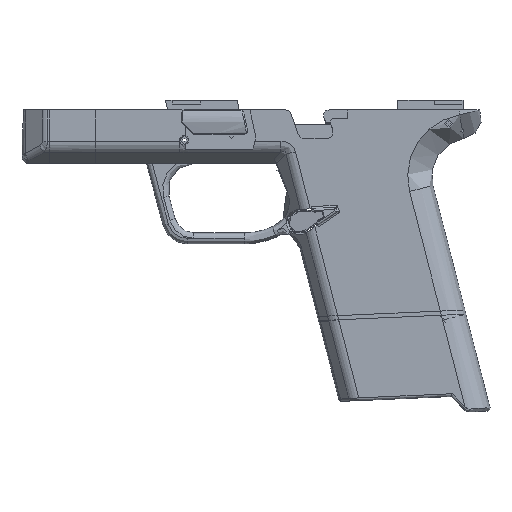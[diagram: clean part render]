
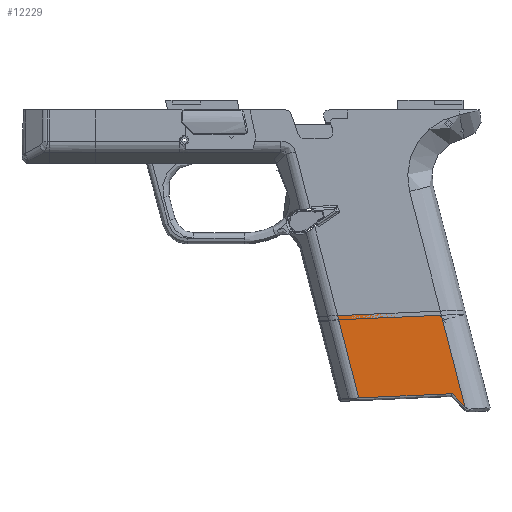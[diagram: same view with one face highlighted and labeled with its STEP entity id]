
A CAD part, left-side view. The second image highlights one B-rep face of the part: STEP entity #12229.
In plain terms, the highlighted face is planar.
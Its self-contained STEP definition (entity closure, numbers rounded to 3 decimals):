
#959=PLANE('',#13436);
#1609=FACE_OUTER_BOUND('',#2307,.T.);
#2307=EDGE_LOOP('',(#11234,#11235,#11236,#11237,#11238));
#3367=LINE('',#23857,#4460);
#3374=LINE('',#23978,#4467);
#3386=LINE('',#24009,#4479);
#3387=LINE('',#24013,#4480);
#3388=LINE('',#24014,#4481);
#4460=VECTOR('',#16590,10.);
#4467=VECTOR('',#16637,10.);
#4479=VECTOR('',#16671,10.);
#4480=VECTOR('',#16676,10.);
#4481=VECTOR('',#16677,10.);
#5935=VERTEX_POINT('',#23689);
#5946=VERTEX_POINT('',#23856);
#5960=VERTEX_POINT('',#23973);
#5968=VERTEX_POINT('',#24008);
#5969=VERTEX_POINT('',#24012);
#7700=EDGE_CURVE('',#5935,#5946,#3367,.T.);
#7723=EDGE_CURVE('',#5946,#5960,#3374,.T.);
#7738=EDGE_CURVE('',#5968,#5960,#3386,.T.);
#7740=EDGE_CURVE('',#5969,#5935,#3387,.T.);
#7741=EDGE_CURVE('',#5969,#5968,#3388,.T.);
#11234=ORIENTED_EDGE('',*,*,#7723,.F.);
#11235=ORIENTED_EDGE('',*,*,#7700,.F.);
#11236=ORIENTED_EDGE('',*,*,#7740,.F.);
#11237=ORIENTED_EDGE('',*,*,#7741,.T.);
#11238=ORIENTED_EDGE('',*,*,#7738,.T.);
#12229=ADVANCED_FACE('',(#1609),#959,.T.);
#13436=AXIS2_PLACEMENT_3D('',#24011,#16674,#16675);
#16590=DIRECTION('',(0.,0.697,-0.717));
#16637=DIRECTION('',(0.,0.999,0.044));
#16671=DIRECTION('',(0.,-0.249,0.969));
#16674=DIRECTION('center_axis',(1.,0.,0.));
#16675=DIRECTION('ref_axis',(0.,0.999,0.044));
#16676=DIRECTION('',(0.,-0.249,0.969));
#16677=DIRECTION('',(0.,0.999,0.044));
#23689=CARTESIAN_POINT('',(22.175,-83.249,100.107));
#23856=CARTESIAN_POINT('',(22.175,-78.67,95.402));
#23857=CARTESIAN_POINT('',(22.175,-73.025,89.603));
#23973=CARTESIAN_POINT('',(22.175,-44.727,96.906));
#23978=CARTESIAN_POINT('',(22.175,-44.598,96.911));
#24008=CARTESIAN_POINT('',(22.175,-37.062,67.087));
#24009=CARTESIAN_POINT('',(22.175,-37.062,67.087));
#24011=CARTESIAN_POINT('Origin',(22.175,-74.337,65.435));
#24012=CARTESIAN_POINT('',(22.175,-74.337,65.435));
#24013=CARTESIAN_POINT('',(22.175,-74.337,65.435));
#24014=CARTESIAN_POINT('',(22.175,-40.4,66.939));
